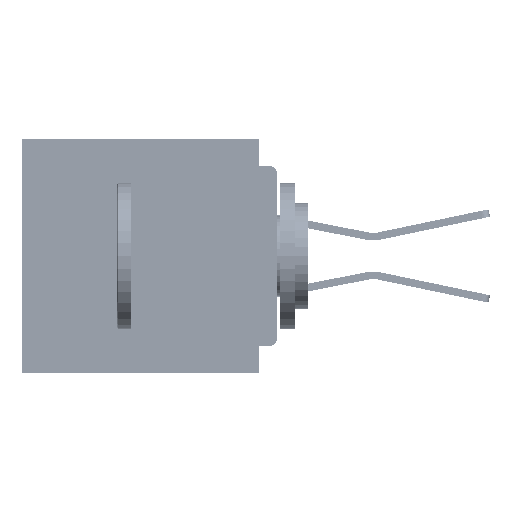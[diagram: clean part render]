
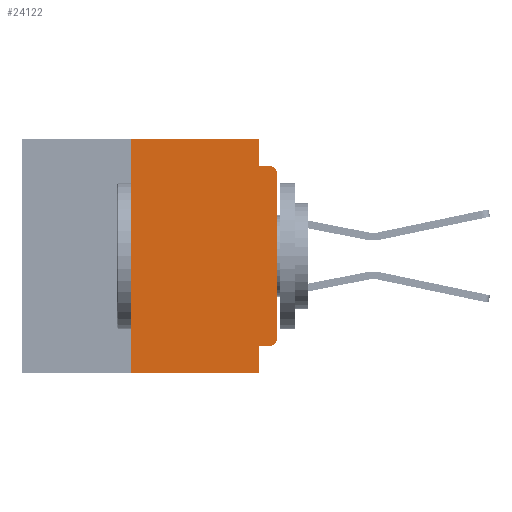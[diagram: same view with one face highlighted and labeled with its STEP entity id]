
A CAD part, left-side view. The second image highlights one B-rep face of the part: STEP entity #24122.
In plain terms, the highlighted planar face has unit normal (-1, 0, 0).
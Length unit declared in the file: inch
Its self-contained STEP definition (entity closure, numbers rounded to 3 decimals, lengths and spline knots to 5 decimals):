
#533 = DIRECTION ( 'NONE',  ( 1., 0., 0. ) ) ;
#551 = ORIENTED_EDGE ( 'NONE', *, *, #10343, .T. ) ;
#1292 = DIRECTION ( 'NONE',  ( 0., 0., 1. ) ) ;
#1436 = AXIS2_PLACEMENT_3D ( 'NONE', #56599, #26766, #61611 ) ;
#1445 = AXIS2_PLACEMENT_3D ( 'NONE', #60658, #533, #35827 ) ;
#3259 = LINE ( 'NONE', #27712, #28577 ) ;
#4326 = CIRCLE ( 'NONE', #1436, 0.015 ) ;
#4612 = CARTESIAN_POINT ( 'NONE',  ( 0., 0., -0.34 ) ) ;
#6589 = CARTESIAN_POINT ( 'NONE',  ( 0., 0.015, -0.06 ) ) ;
#8985 = CARTESIAN_POINT ( 'NONE',  ( 0., 0., -0.355 ) ) ;
#9123 = EDGE_CURVE ( 'NONE', #12952, #63769, #50058, .T. ) ;
#10343 = EDGE_CURVE ( 'NONE', #59926, #16360, #4326, .T. ) ;
#11328 = CARTESIAN_POINT ( 'NONE',  ( 0., 0.031, -0.4 ) ) ;
#11388 = VECTOR ( 'NONE', #32084, 39.37008 ) ;
#11706 = DIRECTION ( 'NONE',  ( 0., 0., -1. ) ) ;
#12952 = VERTEX_POINT ( 'NONE', #34941 ) ;
#13566 = VERTEX_POINT ( 'NONE', #59449 ) ;
#14079 = DIRECTION ( 'NONE',  ( 0., 1., 0. ) ) ;
#16360 = VERTEX_POINT ( 'NONE', #4612 ) ;
#17327 = LINE ( 'NONE', #11328, #55569 ) ;
#18333 = ORIENTED_EDGE ( 'NONE', *, *, #50621, .T. ) ;
#19044 = CARTESIAN_POINT ( 'NONE',  ( 0., 0.031, 0. ) ) ;
#21182 = ORIENTED_EDGE ( 'NONE', *, *, #32906, .F. ) ;
#21680 = ORIENTED_EDGE ( 'NONE', *, *, #26876, .F. ) ;
#22320 = CARTESIAN_POINT ( 'NONE',  ( 0., 0.437, -0.4 ) ) ;
#22451 = CARTESIAN_POINT ( 'NONE',  ( 0., 0.031, -0.4 ) ) ;
#23227 = ORIENTED_EDGE ( 'NONE', *, *, #26297, .T. ) ;
#23324 = ORIENTED_EDGE ( 'NONE', *, *, #62491, .F. ) ;
#23525 = VECTOR ( 'NONE', #37178, 39.37008 ) ;
#24122 = ADVANCED_FACE ( 'NONE', ( #60874 ), #30855, .F. ) ;
#24528 = CARTESIAN_POINT ( 'NONE',  ( 0., 0.437, 0. ) ) ;
#24658 = VERTEX_POINT ( 'NONE', #50595 ) ;
#24813 = LINE ( 'NONE', #61898, #11388 ) ;
#25746 = VECTOR ( 'NONE', #1292, 39.37008 ) ;
#25779 = VERTEX_POINT ( 'NONE', #19044 ) ;
#26297 = EDGE_CURVE ( 'NONE', #16360, #37079, #24813, .T. ) ;
#26766 = DIRECTION ( 'NONE',  ( -1., 0., 0. ) ) ;
#26876 = EDGE_CURVE ( 'NONE', #12952, #13566, #39054, .T. ) ;
#27712 = CARTESIAN_POINT ( 'NONE',  ( 0., 0., -0.045 ) ) ;
#28577 = VECTOR ( 'NONE', #52547, 39.37008 ) ;
#28888 = ORIENTED_EDGE ( 'NONE', *, *, #9123, .T. ) ;
#30247 = CARTESIAN_POINT ( 'NONE',  ( 0., 0.031, 0. ) ) ;
#30855 = PLANE ( 'NONE',  #1445 ) ;
#32084 = DIRECTION ( 'NONE',  ( 0., 0., 1. ) ) ;
#32906 = EDGE_CURVE ( 'NONE', #59926, #40916, #35514, .T. ) ;
#34941 = CARTESIAN_POINT ( 'NONE',  ( 0., 0.25, -0.4 ) ) ;
#35514 = LINE ( 'NONE', #8985, #48769 ) ;
#35827 = DIRECTION ( 'NONE',  ( 0., 0., -1. ) ) ;
#36901 = CARTESIAN_POINT ( 'NONE',  ( 0., 0., -0.06 ) ) ;
#37079 = VERTEX_POINT ( 'NONE', #36901 ) ;
#37178 = DIRECTION ( 'NONE',  ( 0., -1., 0. ) ) ;
#37260 = CIRCLE ( 'NONE', #43633, 0.015 ) ;
#38246 = EDGE_CURVE ( 'NONE', #13566, #25779, #52783, .T. ) ;
#38450 = CARTESIAN_POINT ( 'NONE',  ( 0., 0.015, -0.045 ) ) ;
#39054 = LINE ( 'NONE', #41402, #25746 ) ;
#40294 = DIRECTION ( 'NONE',  ( 0., 0., -1. ) ) ;
#40916 = VERTEX_POINT ( 'NONE', #59298 ) ;
#41402 = CARTESIAN_POINT ( 'NONE',  ( 0., 0.25, -0.4 ) ) ;
#41769 = DIRECTION ( 'NONE',  ( -1., 0., 0. ) ) ;
#43633 = AXIS2_PLACEMENT_3D ( 'NONE', #6589, #41769, #11706 ) ;
#43847 = ORIENTED_EDGE ( 'NONE', *, *, #38246, .F. ) ;
#44205 = DIRECTION ( 'NONE',  ( 0., -1., 0. ) ) ;
#46162 = CARTESIAN_POINT ( 'NONE',  ( 0., 0.015, -0.355 ) ) ;
#46312 = VERTEX_POINT ( 'NONE', #38450 ) ;
#46406 = DIRECTION ( 'NONE',  ( 0., 0., -1. ) ) ;
#48769 = VECTOR ( 'NONE', #14079, 39.37008 ) ;
#50058 = LINE ( 'NONE', #22320, #23525 ) ;
#50435 = EDGE_CURVE ( 'NONE', #25779, #24658, #62967, .T. ) ;
#50595 = CARTESIAN_POINT ( 'NONE',  ( 0., 0.031, -0.045 ) ) ;
#50621 = EDGE_CURVE ( 'NONE', #37079, #46312, #37260, .T. ) ;
#51427 = EDGE_CURVE ( 'NONE', #24658, #46312, #3259, .T. ) ;
#52547 = DIRECTION ( 'NONE',  ( 0., -1., 0. ) ) ;
#52783 = LINE ( 'NONE', #24528, #64416 ) ;
#54981 = EDGE_LOOP ( 'NONE', ( #23227, #18333, #64784, #58816, #43847, #21680, #28888, #23324, #21182, #551 ) ) ;
#55569 = VECTOR ( 'NONE', #46406, 39.37008 ) ;
#56599 = CARTESIAN_POINT ( 'NONE',  ( 0., 0.015, -0.34 ) ) ;
#58816 = ORIENTED_EDGE ( 'NONE', *, *, #50435, .F. ) ;
#59298 = CARTESIAN_POINT ( 'NONE',  ( 0., 0.031, -0.355 ) ) ;
#59449 = CARTESIAN_POINT ( 'NONE',  ( 0., 0.25, 0. ) ) ;
#59926 = VERTEX_POINT ( 'NONE', #46162 ) ;
#60658 = CARTESIAN_POINT ( 'NONE',  ( 0., 0.437, 0. ) ) ;
#60874 = FACE_OUTER_BOUND ( 'NONE', #54981, .T. ) ;
#61430 = VECTOR ( 'NONE', #40294, 39.37008 ) ;
#61611 = DIRECTION ( 'NONE',  ( 0., 0., -1. ) ) ;
#61898 = CARTESIAN_POINT ( 'NONE',  ( 0., 0., 0. ) ) ;
#62491 = EDGE_CURVE ( 'NONE', #40916, #63769, #17327, .T. ) ;
#62967 = LINE ( 'NONE', #30247, #61430 ) ;
#63769 = VERTEX_POINT ( 'NONE', #22451 ) ;
#64416 = VECTOR ( 'NONE', #44205, 39.37008 ) ;
#64784 = ORIENTED_EDGE ( 'NONE', *, *, #51427, .F. ) ;
